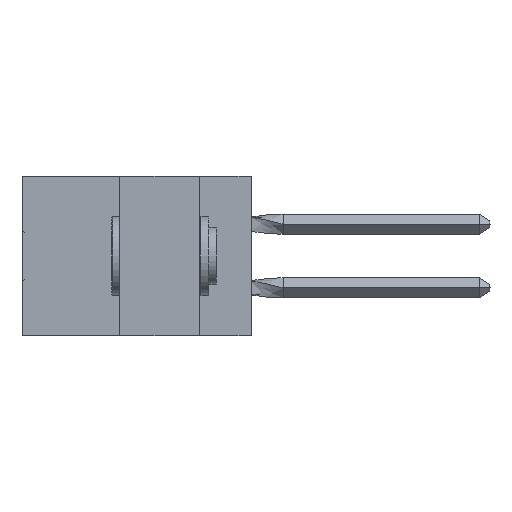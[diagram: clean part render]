
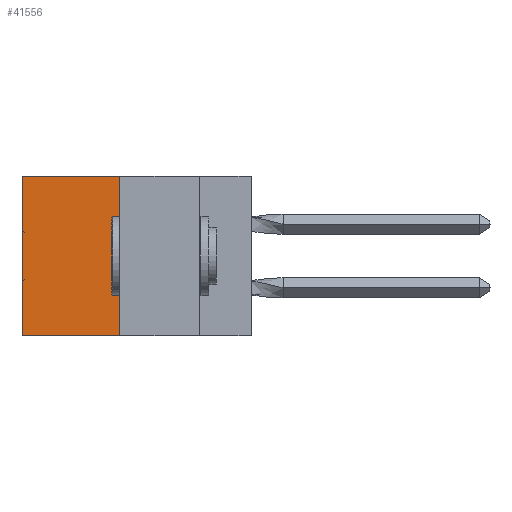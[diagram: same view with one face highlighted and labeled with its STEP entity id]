
A CAD part, left-side view. The second image highlights one B-rep face of the part: STEP entity #41556.
In plain terms, the highlighted planar face has unit normal (-1, 0, 0).
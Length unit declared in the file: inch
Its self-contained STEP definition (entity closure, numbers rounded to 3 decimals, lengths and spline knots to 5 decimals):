
#2443 = CARTESIAN_POINT ( 'NONE',  ( 0.305, 0.413, 0. ) ) ;
#2926 = CARTESIAN_POINT ( 'NONE',  ( 0.305, 0.72, -0.5 ) ) ;
#3197 = ORIENTED_EDGE ( 'NONE', *, *, #45952, .F. ) ;
#6994 = CARTESIAN_POINT ( 'NONE',  ( 0.305, 0.413, -0.5 ) ) ;
#8504 = EDGE_CURVE ( 'NONE', #47598, #19848, #43836, .T. ) ;
#10699 = DIRECTION ( 'NONE',  ( 0., 0., -1. ) ) ;
#11361 = PLANE ( 'NONE',  #41508 ) ;
#11980 = VERTEX_POINT ( 'NONE', #15784 ) ;
#13807 = EDGE_CURVE ( 'NONE', #11980, #19848, #33614, .T. ) ;
#14752 = ORIENTED_EDGE ( 'NONE', *, *, #30951, .T. ) ;
#15338 = CARTESIAN_POINT ( 'NONE',  ( 0.305, 0.72, -0.5 ) ) ;
#15784 = CARTESIAN_POINT ( 'NONE',  ( 0.305, 0.413, -0.5 ) ) ;
#18011 = VECTOR ( 'NONE', #28660, 39.37008 ) ;
#19379 = EDGE_LOOP ( 'NONE', ( #38748, #42881, #3197, #14752 ) ) ;
#19848 = VERTEX_POINT ( 'NONE', #2926 ) ;
#20355 = VECTOR ( 'NONE', #51366, 39.37008 ) ;
#22877 = VECTOR ( 'NONE', #46187, 39.37008 ) ;
#25750 = VERTEX_POINT ( 'NONE', #2443 ) ;
#28166 = DIRECTION ( 'NONE',  ( 0., 0., -1. ) ) ;
#28660 = DIRECTION ( 'NONE',  ( 0., 1., 0. ) ) ;
#30951 = EDGE_CURVE ( 'NONE', #25750, #47598, #32575, .T. ) ;
#31189 = FACE_OUTER_BOUND ( 'NONE', #19379, .T. ) ;
#32575 = LINE ( 'NONE', #44806, #18011 ) ;
#33614 = LINE ( 'NONE', #33724, #22877 ) ;
#33724 = CARTESIAN_POINT ( 'NONE',  ( 0.305, 0.413, -0.5 ) ) ;
#36521 = CARTESIAN_POINT ( 'NONE',  ( 0.305, 0.72, 0. ) ) ;
#38748 = ORIENTED_EDGE ( 'NONE', *, *, #8504, .T. ) ;
#39819 = VECTOR ( 'NONE', #10699, 39.37008 ) ;
#39877 = DIRECTION ( 'NONE',  ( 1., 0., 0. ) ) ;
#41508 = AXIS2_PLACEMENT_3D ( 'NONE', #43781, #39877, #28166 ) ;
#41556 = ADVANCED_FACE ( 'NONE', ( #31189 ), #11361, .F. ) ;
#42881 = ORIENTED_EDGE ( 'NONE', *, *, #13807, .F. ) ;
#43781 = CARTESIAN_POINT ( 'NONE',  ( 0.305, 0.413, -0.5 ) ) ;
#43836 = LINE ( 'NONE', #15338, #20355 ) ;
#44806 = CARTESIAN_POINT ( 'NONE',  ( 0.305, 0.413, 0. ) ) ;
#45952 = EDGE_CURVE ( 'NONE', #25750, #11980, #50618, .T. ) ;
#46187 = DIRECTION ( 'NONE',  ( 0., 1., 0. ) ) ;
#47598 = VERTEX_POINT ( 'NONE', #36521 ) ;
#50618 = LINE ( 'NONE', #6994, #39819 ) ;
#51366 = DIRECTION ( 'NONE',  ( 0., 0., -1. ) ) ;
